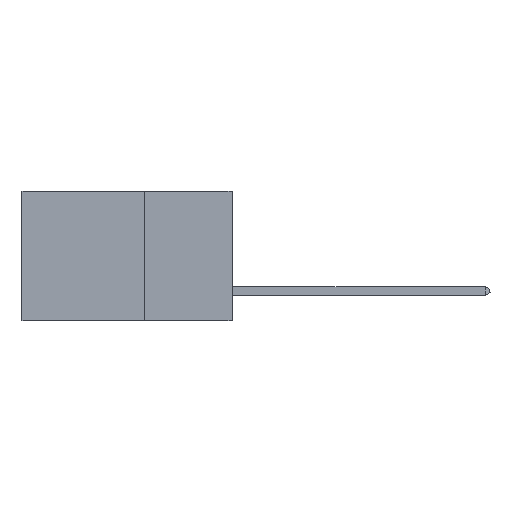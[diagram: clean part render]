
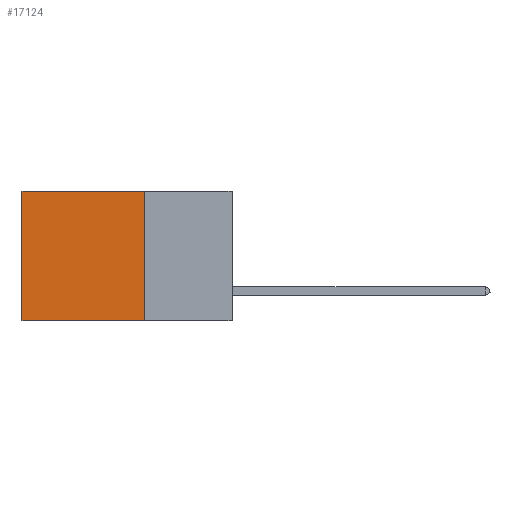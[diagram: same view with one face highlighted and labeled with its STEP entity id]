
A CAD part, left-side view. The second image highlights one B-rep face of the part: STEP entity #17124.
In plain terms, the highlighted planar face has unit normal (-1, 0, 0).
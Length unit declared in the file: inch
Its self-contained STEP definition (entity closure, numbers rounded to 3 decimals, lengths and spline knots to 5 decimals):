
#458 = AXIS2_PLACEMENT_3D ( 'NONE', #8427, #654, #19251 ) ;
#459 = EDGE_LOOP ( 'NONE', ( #20272, #3855, #9583, #18837 ) ) ;
#521 = VERTEX_POINT ( 'NONE', #17665 ) ;
#579 = LINE ( 'NONE', #8510, #11602 ) ;
#654 = DIRECTION ( 'NONE',  ( 1., 0., 0. ) ) ;
#2467 = EDGE_CURVE ( 'NONE', #19753, #521, #579, .T. ) ;
#2793 = CARTESIAN_POINT ( 'NONE',  ( 0.2875, 0.25, 0. ) ) ;
#3801 = DIRECTION ( 'NONE',  ( 0., 1., 0. ) ) ;
#3855 = ORIENTED_EDGE ( 'NONE', *, *, #2467, .F. ) ;
#5778 = VERTEX_POINT ( 'NONE', #16009 ) ;
#5814 = EDGE_CURVE ( 'NONE', #5778, #19753, #18978, .T. ) ;
#6112 = VECTOR ( 'NONE', #9807, 39.37008 ) ;
#8297 = CARTESIAN_POINT ( 'NONE',  ( 0.2875, 0.6, 0. ) ) ;
#8427 = CARTESIAN_POINT ( 'NONE',  ( 0.2875, 0.25, 0. ) ) ;
#8510 = CARTESIAN_POINT ( 'NONE',  ( 0.2875, 0.25, -0.37 ) ) ;
#8598 = CARTESIAN_POINT ( 'NONE',  ( 0.2875, 0.25, -0.37 ) ) ;
#9397 = VECTOR ( 'NONE', #18995, 39.37008 ) ;
#9583 = ORIENTED_EDGE ( 'NONE', *, *, #5814, .F. ) ;
#9639 = CARTESIAN_POINT ( 'NONE',  ( 0.2875, 0.6, 0. ) ) ;
#9807 = DIRECTION ( 'NONE',  ( 0., 0., -1. ) ) ;
#10091 = VERTEX_POINT ( 'NONE', #9639 ) ;
#11602 = VECTOR ( 'NONE', #3801, 39.37008 ) ;
#12361 = FACE_OUTER_BOUND ( 'NONE', #459, .T. ) ;
#12944 = PLANE ( 'NONE',  #458 ) ;
#13754 = LINE ( 'NONE', #8297, #6112 ) ;
#14573 = CARTESIAN_POINT ( 'NONE',  ( 0.2875, 0.25, 0. ) ) ;
#14916 = EDGE_CURVE ( 'NONE', #10091, #521, #13754, .T. ) ;
#16009 = CARTESIAN_POINT ( 'NONE',  ( 0.2875, 0.25, 0. ) ) ;
#17124 = ADVANCED_FACE ( 'NONE', ( #12361 ), #12944, .F. ) ;
#17665 = CARTESIAN_POINT ( 'NONE',  ( 0.2875, 0.6, -0.37 ) ) ;
#18837 = ORIENTED_EDGE ( 'NONE', *, *, #20215, .T. ) ;
#18978 = LINE ( 'NONE', #2793, #9397 ) ;
#18995 = DIRECTION ( 'NONE',  ( 0., 0., -1. ) ) ;
#19053 = VECTOR ( 'NONE', #19316, 39.37008 ) ;
#19251 = DIRECTION ( 'NONE',  ( 0., 0., -1. ) ) ;
#19308 = LINE ( 'NONE', #14573, #19053 ) ;
#19316 = DIRECTION ( 'NONE',  ( 0., 1., 0. ) ) ;
#19753 = VERTEX_POINT ( 'NONE', #8598 ) ;
#20215 = EDGE_CURVE ( 'NONE', #5778, #10091, #19308, .T. ) ;
#20272 = ORIENTED_EDGE ( 'NONE', *, *, #14916, .T. ) ;
